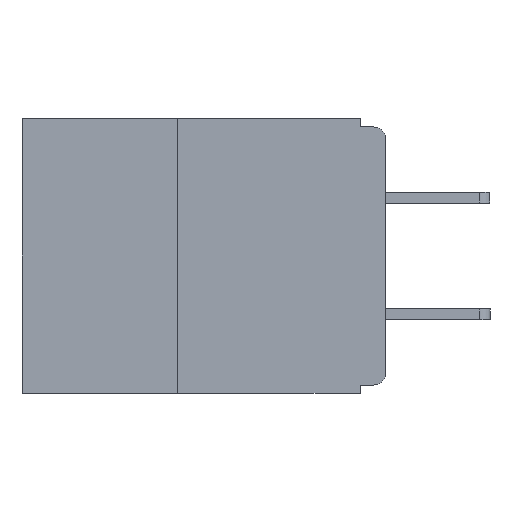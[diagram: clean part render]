
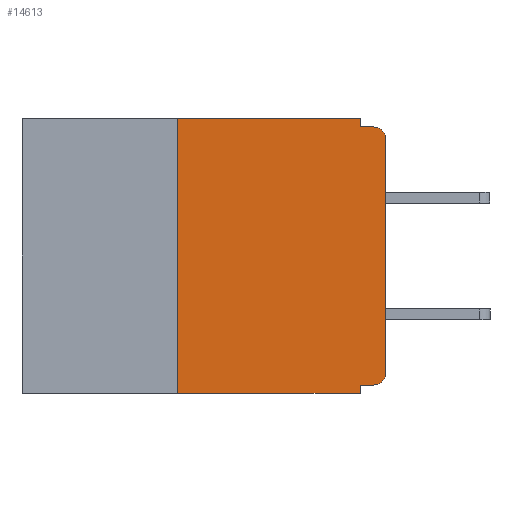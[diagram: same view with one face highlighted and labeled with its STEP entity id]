
A CAD part, left-side view. The second image highlights one B-rep face of the part: STEP entity #14613.
In plain terms, the highlighted planar face has unit normal (-1, 0, 0).
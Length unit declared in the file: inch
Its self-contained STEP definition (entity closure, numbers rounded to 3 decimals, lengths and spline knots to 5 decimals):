
#14 = CIRCLE ( 'NONE', #6609, 0.015 ) ;
#536 = DIRECTION ( 'NONE',  ( 0., 0., 1. ) ) ;
#660 = DIRECTION ( 'NONE',  ( 0., 0., -1. ) ) ;
#766 = CARTESIAN_POINT ( 'NONE',  ( 0., 0.031, 0. ) ) ;
#825 = DIRECTION ( 'NONE',  ( 0., 0., -1. ) ) ;
#1151 = VERTEX_POINT ( 'NONE', #7353 ) ;
#1196 = ORIENTED_EDGE ( 'NONE', *, *, #6315, .F. ) ;
#1386 = DIRECTION ( 'NONE',  ( 0., 0., -1. ) ) ;
#1401 = LINE ( 'NONE', #10846, #6545 ) ;
#1487 = LINE ( 'NONE', #17391, #14477 ) ;
#1684 = AXIS2_PLACEMENT_3D ( 'NONE', #21513, #11643, #1386 ) ;
#2048 = DIRECTION ( 'NONE',  ( 0., -1., 0. ) ) ;
#2359 = LINE ( 'NONE', #18784, #15254 ) ;
#3111 = DIRECTION ( 'NONE',  ( 0., 0., -1. ) ) ;
#3134 = AXIS2_PLACEMENT_3D ( 'NONE', #21023, #11124, #825 ) ;
#3415 = VERTEX_POINT ( 'NONE', #13892 ) ;
#3754 = EDGE_CURVE ( 'NONE', #17276, #9853, #11518, .T. ) ;
#4207 = VECTOR ( 'NONE', #3111, 39.37008 ) ;
#4385 = EDGE_CURVE ( 'NONE', #8096, #12031, #21051, .T. ) ;
#4749 = CARTESIAN_POINT ( 'NONE',  ( 0., 0.015, -0.025 ) ) ;
#4772 = ORIENTED_EDGE ( 'NONE', *, *, #9226, .T. ) ;
#6086 = FACE_OUTER_BOUND ( 'NONE', #21106, .T. ) ;
#6217 = EDGE_CURVE ( 'NONE', #3415, #8096, #1487, .T. ) ;
#6315 = EDGE_CURVE ( 'NONE', #12031, #20645, #20951, .T. ) ;
#6442 = DIRECTION ( 'NONE',  ( 0., 0., -1. ) ) ;
#6545 = VECTOR ( 'NONE', #536, 39.37008 ) ;
#6609 = AXIS2_PLACEMENT_3D ( 'NONE', #4749, #16476, #6442 ) ;
#7119 = VERTEX_POINT ( 'NONE', #8539 ) ;
#7154 = CARTESIAN_POINT ( 'NONE',  ( 0., 0.437, -0.33 ) ) ;
#7353 = CARTESIAN_POINT ( 'NONE',  ( 0., 0.25, -0.33 ) ) ;
#7548 = VECTOR ( 'NONE', #9262, 39.37008 ) ;
#7720 = PLANE ( 'NONE',  #3134 ) ;
#7798 = VECTOR ( 'NONE', #660, 39.37008 ) ;
#8096 = VERTEX_POINT ( 'NONE', #9843 ) ;
#8459 = VERTEX_POINT ( 'NONE', #15768 ) ;
#8468 = EDGE_CURVE ( 'NONE', #21516, #8459, #1401, .T. ) ;
#8539 = CARTESIAN_POINT ( 'NONE',  ( 0., 0.031, -0.33 ) ) ;
#8718 = LINE ( 'NONE', #21435, #4207 ) ;
#8783 = EDGE_CURVE ( 'NONE', #17276, #21516, #18079, .T. ) ;
#8786 = CARTESIAN_POINT ( 'NONE',  ( 0., 0., -0.305 ) ) ;
#9226 = EDGE_CURVE ( 'NONE', #8459, #20645, #14, .T. ) ;
#9255 = EDGE_CURVE ( 'NONE', #9853, #7119, #8718, .T. ) ;
#9262 = DIRECTION ( 'NONE',  ( 0., 1., 0. ) ) ;
#9266 = CARTESIAN_POINT ( 'NONE',  ( 0., 0., -0.32 ) ) ;
#9843 = CARTESIAN_POINT ( 'NONE',  ( 0., 0.031, 0. ) ) ;
#9853 = VERTEX_POINT ( 'NONE', #11464 ) ;
#10846 = CARTESIAN_POINT ( 'NONE',  ( 0., 0., 0. ) ) ;
#11124 = DIRECTION ( 'NONE',  ( 1., 0., 0. ) ) ;
#11410 = ORIENTED_EDGE ( 'NONE', *, *, #4385, .F. ) ;
#11464 = CARTESIAN_POINT ( 'NONE',  ( 0., 0.031, -0.32 ) ) ;
#11518 = LINE ( 'NONE', #9266, #7548 ) ;
#11643 = DIRECTION ( 'NONE',  ( -1., 0., 0. ) ) ;
#11920 = ORIENTED_EDGE ( 'NONE', *, *, #6217, .F. ) ;
#12031 = VERTEX_POINT ( 'NONE', #16270 ) ;
#12165 = VECTOR ( 'NONE', #16498, 39.37008 ) ;
#12951 = ORIENTED_EDGE ( 'NONE', *, *, #18625, .T. ) ;
#13892 = CARTESIAN_POINT ( 'NONE',  ( 0., 0.25, 0. ) ) ;
#14477 = VECTOR ( 'NONE', #17339, 39.37008 ) ;
#14487 = ORIENTED_EDGE ( 'NONE', *, *, #3754, .F. ) ;
#14613 = ADVANCED_FACE ( 'NONE', ( #6086 ), #7720, .F. ) ;
#15254 = VECTOR ( 'NONE', #17232, 39.37008 ) ;
#15768 = CARTESIAN_POINT ( 'NONE',  ( 0., 0., -0.025 ) ) ;
#16148 = VECTOR ( 'NONE', #2048, 39.37008 ) ;
#16270 = CARTESIAN_POINT ( 'NONE',  ( 0., 0.031, -0.01 ) ) ;
#16319 = ORIENTED_EDGE ( 'NONE', *, *, #21556, .F. ) ;
#16476 = DIRECTION ( 'NONE',  ( -1., 0., 0. ) ) ;
#16498 = DIRECTION ( 'NONE',  ( 0., -1., 0. ) ) ;
#16525 = CARTESIAN_POINT ( 'NONE',  ( 0., 0., -0.01 ) ) ;
#17082 = CARTESIAN_POINT ( 'NONE',  ( 0., 0.015, -0.32 ) ) ;
#17232 = DIRECTION ( 'NONE',  ( 0., 0., 1. ) ) ;
#17276 = VERTEX_POINT ( 'NONE', #17082 ) ;
#17339 = DIRECTION ( 'NONE',  ( 0., -1., 0. ) ) ;
#17391 = CARTESIAN_POINT ( 'NONE',  ( 0., 0.437, 0. ) ) ;
#17632 = ORIENTED_EDGE ( 'NONE', *, *, #8468, .T. ) ;
#18079 = CIRCLE ( 'NONE', #1684, 0.015 ) ;
#18625 = EDGE_CURVE ( 'NONE', #1151, #7119, #20535, .T. ) ;
#18784 = CARTESIAN_POINT ( 'NONE',  ( 0., 0.25, -0.33 ) ) ;
#19444 = ORIENTED_EDGE ( 'NONE', *, *, #8783, .T. ) ;
#20535 = LINE ( 'NONE', #7154, #16148 ) ;
#20645 = VERTEX_POINT ( 'NONE', #21288 ) ;
#20951 = LINE ( 'NONE', #16525, #12165 ) ;
#21023 = CARTESIAN_POINT ( 'NONE',  ( 0., 0.437, 0. ) ) ;
#21051 = LINE ( 'NONE', #766, #7798 ) ;
#21106 = EDGE_LOOP ( 'NONE', ( #17632, #4772, #1196, #11410, #11920, #16319, #12951, #21718, #14487, #19444 ) ) ;
#21288 = CARTESIAN_POINT ( 'NONE',  ( 0., 0.015, -0.01 ) ) ;
#21435 = CARTESIAN_POINT ( 'NONE',  ( 0., 0.031, -0.33 ) ) ;
#21513 = CARTESIAN_POINT ( 'NONE',  ( 0., 0.015, -0.305 ) ) ;
#21516 = VERTEX_POINT ( 'NONE', #8786 ) ;
#21556 = EDGE_CURVE ( 'NONE', #1151, #3415, #2359, .T. ) ;
#21718 = ORIENTED_EDGE ( 'NONE', *, *, #9255, .F. ) ;
